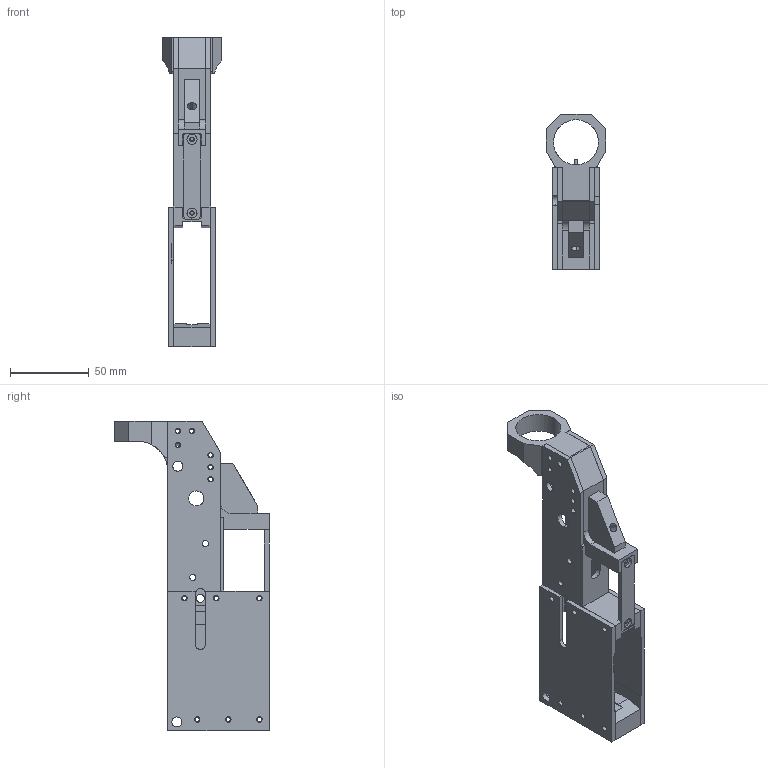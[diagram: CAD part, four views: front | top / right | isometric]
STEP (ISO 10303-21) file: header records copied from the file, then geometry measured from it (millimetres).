
FILE_DESCRIPTION (( 'STEP AP214' ), '1' );
FILE_NAME ('Original_Assembly.STEP', '2015-06-12T14:12:41', ( '' ), ( '' ), 'SwSTEP 2.0', 'SolidWorks 2015', '' );
FILE_SCHEMA (( 'AUTOMOTIVE_DESIGN' ));
Length unit declared in the file: inch
Products named in the file (12): Original_Buffer; Original_Mag_Well_Rear; Original_Mag_Well_Right; Original_Mag_Well_Left; Original_Mag_Well_Front; Original_Side_Left; Original_Fire_Control_Well_Bottom; Original_Side_Right; Original_Assembly; Original_Trigger_Guard; Original_Grip_Part; Original_Buffer_Retainer
Assembly tree (11 placements, depth 2):
  Original_Assembly
    Original_Side_Right
    Original_Fire_Control_Well_Bottom
    Original_Side_Left
    Original_Mag_Well_Front
    Original_Mag_Well_Left
    Original_Mag_Well_Right
    Original_Mag_Well_Rear
    Original_Buffer
    Original_Buffer_Retainer
    Original_Grip_Part
    Original_Trigger_Guard
Bounding box: 37.49 x 98.02 x 196.29 mm (x, y, z)
Volume: 124693.2 mm3; surface area: 75636.1 mm2
Topology: 11 solids, 11 shells, 373 faces, 1035 edges, 688 vertices
Faces by surface type: plane 197, cylinder 176
Entity records: 13052 total; most frequent: CARTESIAN_POINT 2360, DIRECTION 2140, ORIENTED_EDGE 2070, EDGE_CURVE 1035, AXIS2_PLACEMENT_3D 742, VERTEX_POINT 688, VECTOR 656, LINE 656
